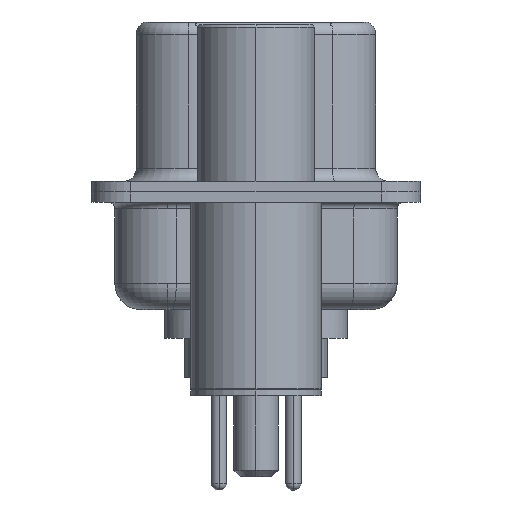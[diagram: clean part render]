
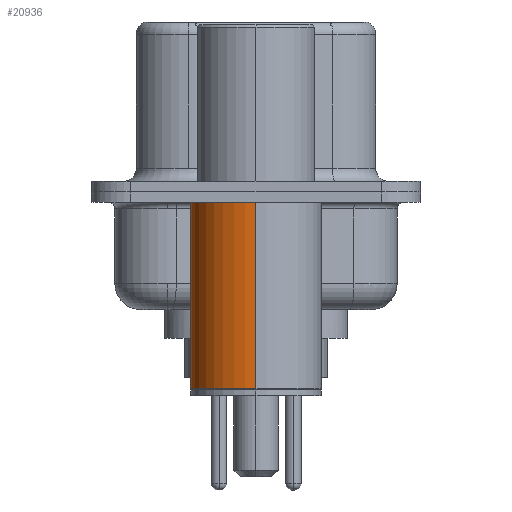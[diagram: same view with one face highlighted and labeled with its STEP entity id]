
A CAD part, left-side view. The second image highlights one B-rep face of the part: STEP entity #20936.
In plain terms, the highlighted cylindrical face has radius 2.5 mm (diameter 5 mm), a partial arc.
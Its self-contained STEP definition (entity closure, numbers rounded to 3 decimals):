
#420 = VERTEX_POINT ( 'NONE', #17787 ) ;
#884 = DIRECTION ( 'NONE',  ( 1., 0., 0. ) ) ;
#982 = CARTESIAN_POINT ( 'NONE',  ( 2.5, 0., 0.581 ) ) ;
#1804 = CARTESIAN_POINT ( 'NONE',  ( 0., 0., -7.525 ) ) ;
#3967 = DIRECTION ( 'NONE',  ( 1., 0., 0. ) ) ;
#4617 = ORIENTED_EDGE ( 'NONE', *, *, #15823, .T. ) ;
#6282 = CARTESIAN_POINT ( 'NONE',  ( -2.5, 0., 0.581 ) ) ;
#7835 = EDGE_LOOP ( 'NONE', ( #11485, #4617, #21065, #17036 ) ) ;
#8500 = LINE ( 'NONE', #6282, #13690 ) ;
#8633 = EDGE_CURVE ( 'NONE', #14492, #20261, #10062, .T. ) ;
#8675 = EDGE_CURVE ( 'NONE', #420, #14492, #25624, .T. ) ;
#10038 = VERTEX_POINT ( 'NONE', #10286 ) ;
#10062 = CIRCLE ( 'NONE', #11276, 2.5 ) ;
#10286 = CARTESIAN_POINT ( 'NONE',  ( -2.5, 0., -7.525 ) ) ;
#11276 = AXIS2_PLACEMENT_3D ( 'NONE', #27316, #14057, #884 ) ;
#11292 = EDGE_CURVE ( 'NONE', #420, #10038, #18368, .T. ) ;
#11485 = ORIENTED_EDGE ( 'NONE', *, *, #11292, .T. ) ;
#11598 = DIRECTION ( 'NONE',  ( 1., 0., 0. ) ) ;
#11944 = DIRECTION ( 'NONE',  ( 0., 0., 1. ) ) ;
#13690 = VECTOR ( 'NONE', #23884, 1000. ) ;
#14057 = DIRECTION ( 'NONE',  ( 0., 0., 1. ) ) ;
#14492 = VERTEX_POINT ( 'NONE', #18424 ) ;
#15723 = CYLINDRICAL_SURFACE ( 'NONE', #17151, 2.5 ) ;
#15823 = EDGE_CURVE ( 'NONE', #10038, #20261, #8500, .T. ) ;
#16378 = AXIS2_PLACEMENT_3D ( 'NONE', #1804, #17214, #3967 ) ;
#16401 = FACE_OUTER_BOUND ( 'NONE', #7835, .T. ) ;
#17036 = ORIENTED_EDGE ( 'NONE', *, *, #8675, .F. ) ;
#17151 = AXIS2_PLACEMENT_3D ( 'NONE', #24831, #22117, #11598 ) ;
#17214 = DIRECTION ( 'NONE',  ( 0., 0., 1. ) ) ;
#17787 = CARTESIAN_POINT ( 'NONE',  ( 2.5, 0., -7.525 ) ) ;
#18368 = CIRCLE ( 'NONE', #16378, 2.5 ) ;
#18424 = CARTESIAN_POINT ( 'NONE',  ( 2.5, 0., -0.4 ) ) ;
#19717 = VECTOR ( 'NONE', #11944, 1000. ) ;
#20261 = VERTEX_POINT ( 'NONE', #23933 ) ;
#20936 = ADVANCED_FACE ( 'NONE', ( #16401 ), #15723, .T. ) ;
#21065 = ORIENTED_EDGE ( 'NONE', *, *, #8633, .F. ) ;
#22117 = DIRECTION ( 'NONE',  ( 0., 0., 1. ) ) ;
#23884 = DIRECTION ( 'NONE',  ( 0., 0., 1. ) ) ;
#23933 = CARTESIAN_POINT ( 'NONE',  ( -2.5, 0., -0.4 ) ) ;
#24831 = CARTESIAN_POINT ( 'NONE',  ( 0., 0., 0.581 ) ) ;
#25624 = LINE ( 'NONE', #982, #19717 ) ;
#27316 = CARTESIAN_POINT ( 'NONE',  ( 0., 0., -0.4 ) ) ;
